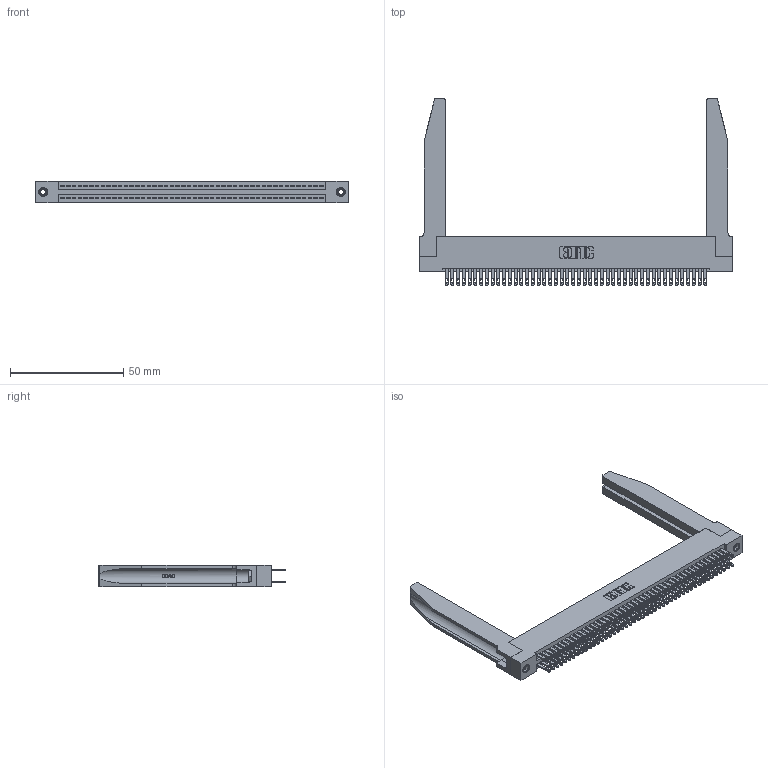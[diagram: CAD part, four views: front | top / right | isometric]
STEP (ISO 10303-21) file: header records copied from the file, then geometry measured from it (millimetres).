
FILE_DESCRIPTION (( 'STEP AP203' ), '1' );
FILE_NAME ('345-092-500-278.STEP', '2019-11-01T17:58:16', ( '' ), ( '' ), 'SwSTEP 2.0', 'SolidWorks 2016', '' );
FILE_SCHEMA (( 'CONFIG_CONTROL_DESIGN' ));
Length unit declared in the file: inch
Products named in the file (5): 345-092-500-278; 345-292-001_345-293-100; 345-250-001_345-250-001-102; 345 Part_Flush Mounting Lugs - 0.156 Dia-TH; 345-220-078_345-220-078
Assembly tree (97 placements, depth 2):
  345-092-500-278
    345 Part_Flush Mounting Lugs - 0.156 Dia-TH
    345-292-001_345-293-100  x92
    345-250-001_345-250-001-102  x2
    345-220-078_345-220-078  x2
Bounding box: 138.07 x 82.47 x 9.4 mm (x, y, z)
Volume: 21501.4 mm3; surface area: 28150.9 mm2
Topology: 97 solids, 97 shells, 4592 faces, 13921 edges, 9270 vertices
Faces by surface type: plane 2706, cylinder 1834, bspline 36, cone 12, torus 4
Entity records: 40224 total; most frequent: CARTESIAN_POINT 7655, ORIENTED_EDGE 6486, DIRECTION 5741, EDGE_CURVE 3243, VECTOR 2829, LINE 2829, VERTEX_POINT 2156, AXIS2_PLACEMENT_3D 1456
